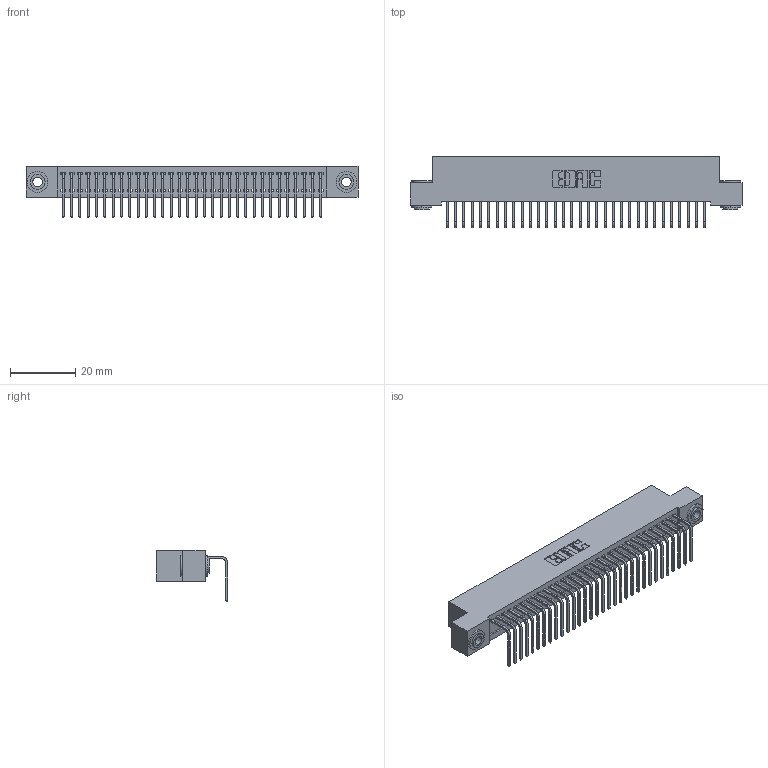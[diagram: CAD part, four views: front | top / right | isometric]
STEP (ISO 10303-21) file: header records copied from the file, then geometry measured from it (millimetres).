
FILE_DESCRIPTION (( 'STEP AP203' ), '1' );
FILE_NAME ('342-032-558-103.STEP', '2019-10-02T11:21:43', ( '' ), ( '' ), 'SwSTEP 2.0', 'SolidWorks 2016', '' );
FILE_SCHEMA (( 'CONFIG_CONTROL_DESIGN' ));
Length unit declared in the file: inch
Products named in the file (4): 342-032-558-103; 342 Part_.156 TH; 345-292-001_558 Tail - 2; 342-250-002_345-250-002-102
Assembly tree (35 placements, depth 2):
  342-032-558-103
    342 Part_.156 TH
    345-292-001_558 Tail - 2  x32
    342-250-002_345-250-002-102  x2
Bounding box: 101.6 x 21.91 x 15.62 mm (x, y, z)
Volume: 9000.9 mm3; surface area: 13862.4 mm2
Topology: 35 solids, 35 shells, 2068 faces, 6199 edges, 4086 vertices
Faces by surface type: plane 1484, cylinder 576, cone 8
Entity records: 21458 total; most frequent: CARTESIAN_POINT 3681, ORIENTED_EDGE 3642, DIRECTION 3159, EDGE_CURVE 1821, LINE 1669, VECTOR 1669, VERTEX_POINT 1210, AXIS2_PLACEMENT_3D 745
